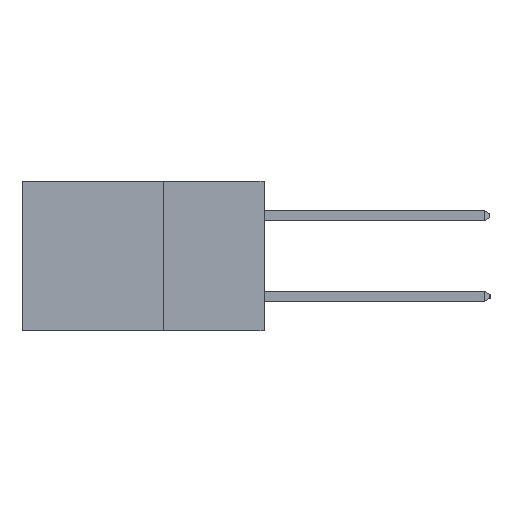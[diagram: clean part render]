
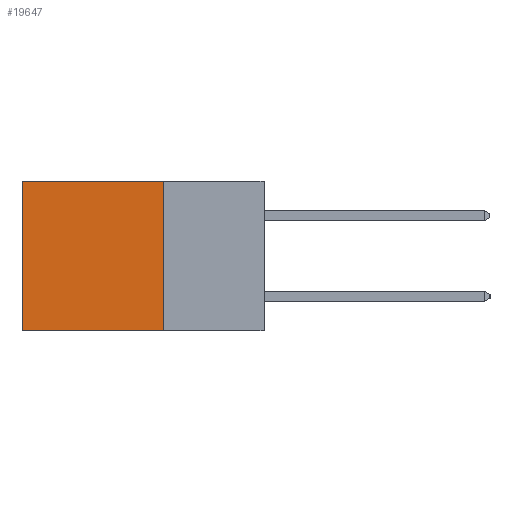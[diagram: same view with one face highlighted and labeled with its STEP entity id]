
A CAD part, left-side view. The second image highlights one B-rep face of the part: STEP entity #19647.
In plain terms, the highlighted planar face has unit normal (-1, 0, 0).
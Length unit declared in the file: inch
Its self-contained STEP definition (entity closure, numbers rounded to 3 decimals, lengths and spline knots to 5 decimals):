
#196 = LINE ( 'NONE', #2393, #13348 ) ;
#638 = CARTESIAN_POINT ( 'NONE',  ( 0.2615, 0.25, -0.37 ) ) ;
#836 = VERTEX_POINT ( 'NONE', #3362 ) ;
#1534 = AXIS2_PLACEMENT_3D ( 'NONE', #18712, #13734, #3465 ) ;
#1704 = VERTEX_POINT ( 'NONE', #638 ) ;
#1744 = PLANE ( 'NONE',  #1534 ) ;
#2393 = CARTESIAN_POINT ( 'NONE',  ( 0.2615, 0.25, -0.37 ) ) ;
#2874 = VERTEX_POINT ( 'NONE', #15489 ) ;
#2991 = ORIENTED_EDGE ( 'NONE', *, *, #19978, .T. ) ;
#3362 = CARTESIAN_POINT ( 'NONE',  ( 0.2615, 0.25, 0. ) ) ;
#3465 = DIRECTION ( 'NONE',  ( 0., 0., -1. ) ) ;
#4114 = DIRECTION ( 'NONE',  ( 0., 0., -1. ) ) ;
#4388 = DIRECTION ( 'NONE',  ( 0., 1., 0. ) ) ;
#5473 = VECTOR ( 'NONE', #21186, 39.37008 ) ;
#6486 = LINE ( 'NONE', #7867, #15065 ) ;
#7149 = CARTESIAN_POINT ( 'NONE',  ( 0.2615, 0.6, -0.37 ) ) ;
#7867 = CARTESIAN_POINT ( 'NONE',  ( 0.2615, 0.25, -0.37 ) ) ;
#8891 = DIRECTION ( 'NONE',  ( 0., 0., -1. ) ) ;
#9918 = EDGE_CURVE ( 'NONE', #1704, #2874, #6486, .T. ) ;
#9986 = VERTEX_POINT ( 'NONE', #14878 ) ;
#11950 = LINE ( 'NONE', #7149, #19780 ) ;
#12211 = EDGE_CURVE ( 'NONE', #836, #1704, #196, .T. ) ;
#13348 = VECTOR ( 'NONE', #4114, 39.37008 ) ;
#13449 = EDGE_CURVE ( 'NONE', #9986, #2874, #11950, .T. ) ;
#13734 = DIRECTION ( 'NONE',  ( 1., 0., 0. ) ) ;
#14127 = ORIENTED_EDGE ( 'NONE', *, *, #9918, .F. ) ;
#14571 = LINE ( 'NONE', #19543, #5473 ) ;
#14878 = CARTESIAN_POINT ( 'NONE',  ( 0.2615, 0.6, 0. ) ) ;
#15065 = VECTOR ( 'NONE', #4388, 39.37008 ) ;
#15489 = CARTESIAN_POINT ( 'NONE',  ( 0.2615, 0.6, -0.37 ) ) ;
#16893 = ORIENTED_EDGE ( 'NONE', *, *, #12211, .F. ) ;
#16959 = FACE_OUTER_BOUND ( 'NONE', #18684, .T. ) ;
#18684 = EDGE_LOOP ( 'NONE', ( #21914, #14127, #16893, #2991 ) ) ;
#18712 = CARTESIAN_POINT ( 'NONE',  ( 0.2615, 0.25, -0.37 ) ) ;
#19543 = CARTESIAN_POINT ( 'NONE',  ( 0.2615, 0.25, 0. ) ) ;
#19647 = ADVANCED_FACE ( 'NONE', ( #16959 ), #1744, .F. ) ;
#19780 = VECTOR ( 'NONE', #8891, 39.37008 ) ;
#19978 = EDGE_CURVE ( 'NONE', #836, #9986, #14571, .T. ) ;
#21186 = DIRECTION ( 'NONE',  ( 0., 1., 0. ) ) ;
#21914 = ORIENTED_EDGE ( 'NONE', *, *, #13449, .T. ) ;
